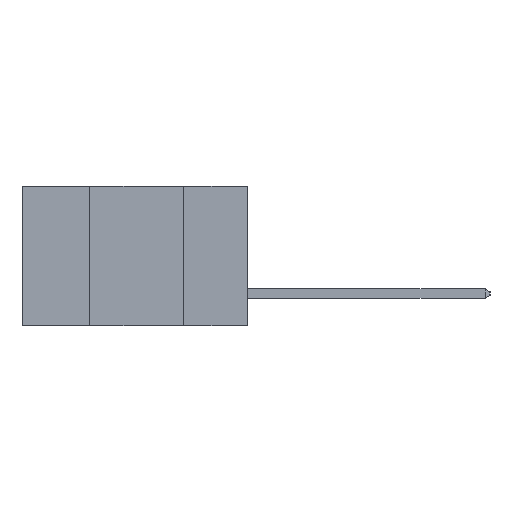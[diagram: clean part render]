
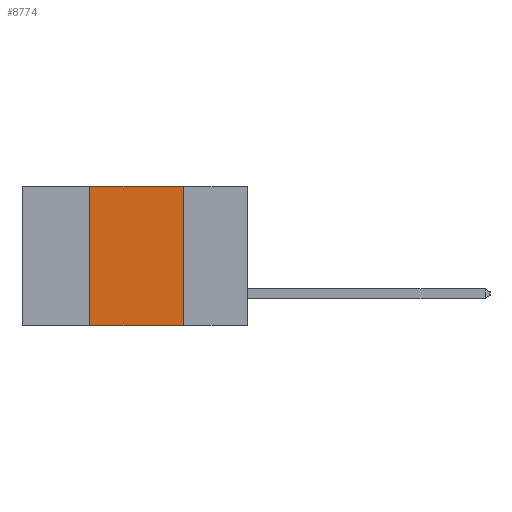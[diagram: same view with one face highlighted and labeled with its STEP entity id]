
A CAD part, left-side view. The second image highlights one B-rep face of the part: STEP entity #8774.
In plain terms, the highlighted planar face has unit normal (-1, 0, 0).
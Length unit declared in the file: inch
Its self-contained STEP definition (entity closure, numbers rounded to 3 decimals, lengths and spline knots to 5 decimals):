
#261 = EDGE_LOOP ( 'NONE', ( #11865, #8382, #10384, #8506 ) ) ;
#279 = DIRECTION ( 'NONE',  ( 1., 0., 0. ) ) ;
#810 = VECTOR ( 'NONE', #7458, 39.37008 ) ;
#963 = VECTOR ( 'NONE', #7477, 39.37008 ) ;
#1121 = LINE ( 'NONE', #4687, #810 ) ;
#1786 = DIRECTION ( 'NONE',  ( 0., -1., 0. ) ) ;
#2260 = CARTESIAN_POINT ( 'NONE',  ( 0., 0.6, 0. ) ) ;
#2805 = CARTESIAN_POINT ( 'NONE',  ( 0., 0.42, 0. ) ) ;
#2999 = CARTESIAN_POINT ( 'NONE',  ( 0., 0.42, -0.37 ) ) ;
#3433 = VECTOR ( 'NONE', #10212, 39.37008 ) ;
#4286 = VERTEX_POINT ( 'NONE', #5777 ) ;
#4687 = CARTESIAN_POINT ( 'NONE',  ( 0., 0.6, 0. ) ) ;
#4992 = EDGE_CURVE ( 'NONE', #5494, #4286, #8509, .T. ) ;
#5494 = VERTEX_POINT ( 'NONE', #8038 ) ;
#5777 = CARTESIAN_POINT ( 'NONE',  ( 0., 0.17, -0.37 ) ) ;
#5804 = CARTESIAN_POINT ( 'NONE',  ( 0., 0.42, -0.37 ) ) ;
#6122 = VERTEX_POINT ( 'NONE', #2805 ) ;
#6156 = PLANE ( 'NONE',  #10256 ) ;
#6506 = CARTESIAN_POINT ( 'NONE',  ( 0., 0.17, -0.37 ) ) ;
#6571 = VECTOR ( 'NONE', #1786, 39.37008 ) ;
#7066 = DIRECTION ( 'NONE',  ( 0., 0., -1. ) ) ;
#7068 = EDGE_CURVE ( 'NONE', #6122, #5494, #1121, .T. ) ;
#7458 = DIRECTION ( 'NONE',  ( 0., -1., 0. ) ) ;
#7477 = DIRECTION ( 'NONE',  ( 0., 0., -1. ) ) ;
#7559 = FACE_OUTER_BOUND ( 'NONE', #261, .T. ) ;
#8038 = CARTESIAN_POINT ( 'NONE',  ( 0., 0.17, 0. ) ) ;
#8382 = ORIENTED_EDGE ( 'NONE', *, *, #7068, .F. ) ;
#8463 = VERTEX_POINT ( 'NONE', #5804 ) ;
#8506 = ORIENTED_EDGE ( 'NONE', *, *, #9071, .T. ) ;
#8509 = LINE ( 'NONE', #6506, #963 ) ;
#8576 = LINE ( 'NONE', #2999, #3433 ) ;
#8774 = ADVANCED_FACE ( 'NONE', ( #7559 ), #6156, .F. ) ;
#8892 = LINE ( 'NONE', #10893, #6571 ) ;
#9071 = EDGE_CURVE ( 'NONE', #8463, #4286, #8892, .T. ) ;
#10212 = DIRECTION ( 'NONE',  ( 0., 0., 1. ) ) ;
#10256 = AXIS2_PLACEMENT_3D ( 'NONE', #2260, #279, #7066 ) ;
#10384 = ORIENTED_EDGE ( 'NONE', *, *, #10898, .F. ) ;
#10893 = CARTESIAN_POINT ( 'NONE',  ( 0., 0.6, -0.37 ) ) ;
#10898 = EDGE_CURVE ( 'NONE', #8463, #6122, #8576, .T. ) ;
#11865 = ORIENTED_EDGE ( 'NONE', *, *, #4992, .F. ) ;
